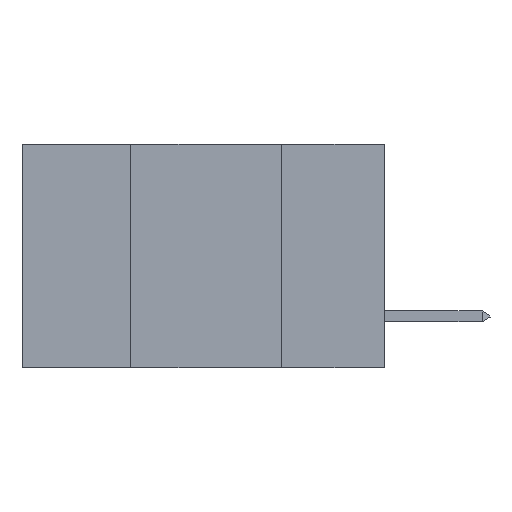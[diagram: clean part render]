
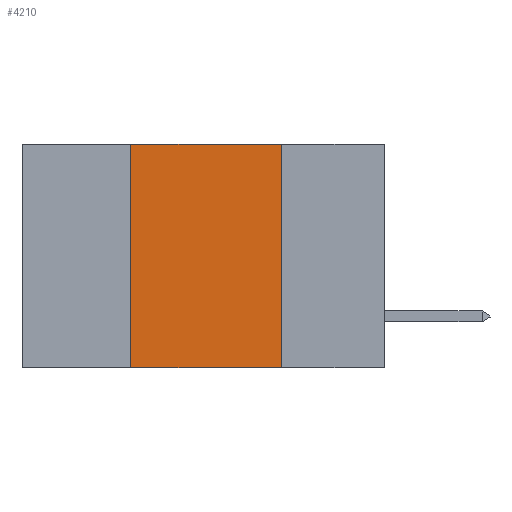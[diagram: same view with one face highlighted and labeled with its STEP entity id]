
A CAD part, left-side view. The second image highlights one B-rep face of the part: STEP entity #4210.
In plain terms, the highlighted planar face has unit normal (-1, 0, 0).
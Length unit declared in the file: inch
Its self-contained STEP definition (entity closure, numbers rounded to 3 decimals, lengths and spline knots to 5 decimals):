
#5 = VECTOR ( 'NONE', #6802, 39.37008 ) ;
#254 = VECTOR ( 'NONE', #2299, 39.37008 ) ;
#338 = EDGE_CURVE ( 'NONE', #938, #6295, #2214, .T. ) ;
#376 = ORIENTED_EDGE ( 'NONE', *, *, #1544, .F. ) ;
#675 = CARTESIAN_POINT ( 'NONE',  ( 0., 0.42, 0. ) ) ;
#938 = VERTEX_POINT ( 'NONE', #5072 ) ;
#1188 = DIRECTION ( 'NONE',  ( 0., -1., 0. ) ) ;
#1544 = EDGE_CURVE ( 'NONE', #6295, #7672, #7483, .T. ) ;
#1682 = EDGE_LOOP ( 'NONE', ( #4221, #376, #10461, #6858 ) ) ;
#2112 = DIRECTION ( 'NONE',  ( 0., 0., -1. ) ) ;
#2214 = LINE ( 'NONE', #8554, #5 ) ;
#2299 = DIRECTION ( 'NONE',  ( 0., -1., 0. ) ) ;
#4210 = ADVANCED_FACE ( 'NONE', ( #6538 ), #4547, .F. ) ;
#4221 = ORIENTED_EDGE ( 'NONE', *, *, #6001, .F. ) ;
#4547 = PLANE ( 'NONE',  #4573 ) ;
#4573 = AXIS2_PLACEMENT_3D ( 'NONE', #5394, #10659, #9827 ) ;
#4839 = CARTESIAN_POINT ( 'NONE',  ( 0., 0.17, 0. ) ) ;
#4869 = EDGE_CURVE ( 'NONE', #938, #7894, #4926, .T. ) ;
#4895 = VECTOR ( 'NONE', #2112, 39.37008 ) ;
#4926 = LINE ( 'NONE', #9594, #10294 ) ;
#5072 = CARTESIAN_POINT ( 'NONE',  ( 0., 0.42, -0.37 ) ) ;
#5394 = CARTESIAN_POINT ( 'NONE',  ( 0., 0.6, 0. ) ) ;
#6001 = EDGE_CURVE ( 'NONE', #7672, #7894, #7006, .T. ) ;
#6295 = VERTEX_POINT ( 'NONE', #675 ) ;
#6538 = FACE_OUTER_BOUND ( 'NONE', #1682, .T. ) ;
#6802 = DIRECTION ( 'NONE',  ( 0., 0., 1. ) ) ;
#6858 = ORIENTED_EDGE ( 'NONE', *, *, #4869, .T. ) ;
#7006 = LINE ( 'NONE', #9754, #4895 ) ;
#7483 = LINE ( 'NONE', #10582, #254 ) ;
#7672 = VERTEX_POINT ( 'NONE', #4839 ) ;
#7894 = VERTEX_POINT ( 'NONE', #7922 ) ;
#7922 = CARTESIAN_POINT ( 'NONE',  ( 0., 0.17, -0.37 ) ) ;
#8554 = CARTESIAN_POINT ( 'NONE',  ( 0., 0.42, 0. ) ) ;
#9594 = CARTESIAN_POINT ( 'NONE',  ( 0., 0.6, -0.37 ) ) ;
#9754 = CARTESIAN_POINT ( 'NONE',  ( 0., 0.17, 0. ) ) ;
#9827 = DIRECTION ( 'NONE',  ( 0., 0., -1. ) ) ;
#10294 = VECTOR ( 'NONE', #1188, 39.37008 ) ;
#10461 = ORIENTED_EDGE ( 'NONE', *, *, #338, .F. ) ;
#10582 = CARTESIAN_POINT ( 'NONE',  ( 0., 0.6, 0. ) ) ;
#10659 = DIRECTION ( 'NONE',  ( 1., 0., 0. ) ) ;
